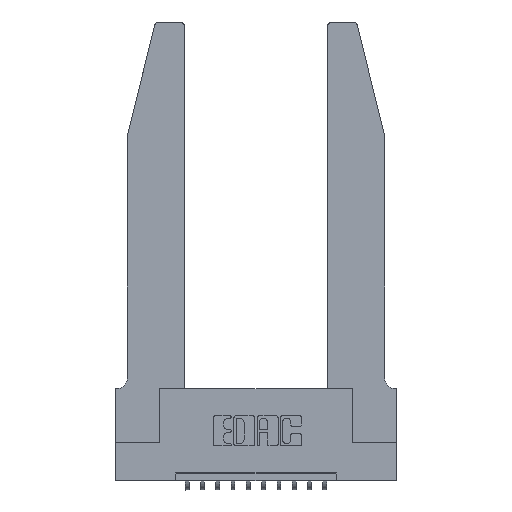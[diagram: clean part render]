
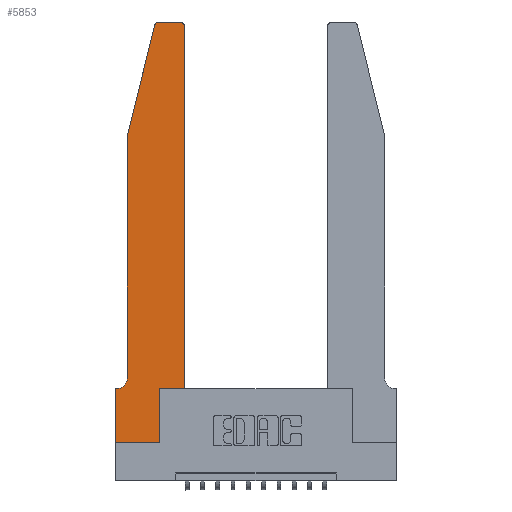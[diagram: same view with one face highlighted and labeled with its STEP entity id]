
A CAD part, top view. The second image highlights one B-rep face of the part: STEP entity #5853.
In plain terms, the highlighted planar face has unit normal (0, 0, 1).
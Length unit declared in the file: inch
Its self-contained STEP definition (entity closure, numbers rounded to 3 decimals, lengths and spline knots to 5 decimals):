
#32 = DIRECTION ( 'NONE',  ( 1., 0., 0. ) ) ;
#38 = ORIENTED_EDGE ( 'NONE', *, *, #14863, .T. ) ;
#209 = VERTEX_POINT ( 'NONE', #15698 ) ;
#236 = PLANE ( 'NONE',  #3552 ) ;
#240 = DIRECTION ( 'NONE',  ( 0., 0., 1. ) ) ;
#488 = CARTESIAN_POINT ( 'NONE',  ( 0.0755, 2., 0.37 ) ) ;
#727 = AXIS2_PLACEMENT_3D ( 'NONE', #13966, #15310, #10030 ) ;
#1046 = EDGE_CURVE ( 'NONE', #7538, #15131, #4470, .T. ) ;
#1056 = ORIENTED_EDGE ( 'NONE', *, *, #11195, .T. ) ;
#1057 = ORIENTED_EDGE ( 'NONE', *, *, #8504, .T. ) ;
#1483 = DIRECTION ( 'NONE',  ( -1., 0., 0. ) ) ;
#1538 = ORIENTED_EDGE ( 'NONE', *, *, #12622, .T. ) ;
#2550 = ORIENTED_EDGE ( 'NONE', *, *, #3011, .T. ) ;
#2638 = DIRECTION ( 'NONE',  ( 0., -1., 0. ) ) ;
#2800 = DIRECTION ( 'NONE',  ( 0., 0., -1. ) ) ;
#2969 = VECTOR ( 'NONE', #8271, 39.37008 ) ;
#3011 = EDGE_CURVE ( 'NONE', #15131, #6401, #12702, .T. ) ;
#3384 = VERTEX_POINT ( 'NONE', #8757 ) ;
#3529 = VECTOR ( 'NONE', #15732, 39.37008 ) ;
#3552 = AXIS2_PLACEMENT_3D ( 'NONE', #10626, #240, #4208 ) ;
#3929 = DIRECTION ( 'NONE',  ( 0., 1., 0. ) ) ;
#3962 = CARTESIAN_POINT ( 'NONE',  ( 0.4205, 2.75, 0.37 ) ) ;
#4182 = CARTESIAN_POINT ( 'NONE',  ( 0., 0., 0.37 ) ) ;
#4208 = DIRECTION ( 'NONE',  ( 1., 0., 0. ) ) ;
#4231 = CARTESIAN_POINT ( 'NONE',  ( 0.25487, 2.72718, 0.37 ) ) ;
#4266 = VECTOR ( 'NONE', #9785, 39.37008 ) ;
#4470 = LINE ( 'NONE', #8400, #4266 ) ;
#4606 = DIRECTION ( 'NONE',  ( 0., -1., 0. ) ) ;
#5055 = ORIENTED_EDGE ( 'NONE', *, *, #6275, .T. ) ;
#5202 = CARTESIAN_POINT ( 'NONE',  ( 0.4205, 2.72, 0.37 ) ) ;
#5614 = CARTESIAN_POINT ( 'NONE',  ( 0.284, 2.75, 0.37 ) ) ;
#5672 = DIRECTION ( 'NONE',  ( -0.239, -0.971, 0. ) ) ;
#5853 = ADVANCED_FACE ( 'NONE', ( #15556 ), #236, .T. ) ;
#5855 = VERTEX_POINT ( 'NONE', #13313 ) ;
#5894 = CARTESIAN_POINT ( 'NONE',  ( 0.0055, 0.35, 0.37 ) ) ;
#5987 = EDGE_CURVE ( 'NONE', #13881, #9811, #12895, .T. ) ;
#6173 = EDGE_CURVE ( 'NONE', #6401, #13881, #13934, .T. ) ;
#6275 = EDGE_CURVE ( 'NONE', #209, #5855, #8270, .T. ) ;
#6278 = EDGE_CURVE ( 'NONE', #13497, #12828, #12287, .T. ) ;
#6327 = VERTEX_POINT ( 'NONE', #5894 ) ;
#6401 = VERTEX_POINT ( 'NONE', #4231 ) ;
#6604 = DIRECTION ( 'NONE',  ( -1., 0., 0. ) ) ;
#7230 = ORIENTED_EDGE ( 'NONE', *, *, #6173, .T. ) ;
#7538 = VERTEX_POINT ( 'NONE', #3962 ) ;
#7610 = CARTESIAN_POINT ( 'NONE',  ( 0.4505, 0.35, 0.37 ) ) ;
#7683 = AXIS2_PLACEMENT_3D ( 'NONE', #10397, #2800, #6604 ) ;
#7750 = LINE ( 'NONE', #13047, #14407 ) ;
#7888 = ORIENTED_EDGE ( 'NONE', *, *, #6278, .T. ) ;
#8023 = CARTESIAN_POINT ( 'NONE',  ( 0.0755, 0.42, 0.37 ) ) ;
#8270 = LINE ( 'NONE', #9878, #13723 ) ;
#8271 = DIRECTION ( 'NONE',  ( 0., 1., 0. ) ) ;
#8400 = CARTESIAN_POINT ( 'NONE',  ( 0.2605, 2.75, 0.37 ) ) ;
#8429 = EDGE_CURVE ( 'NONE', #9811, #6327, #14061, .T. ) ;
#8504 = EDGE_CURVE ( 'NONE', #12828, #3384, #10376, .T. ) ;
#8757 = CARTESIAN_POINT ( 'NONE',  ( 0.2865, 0., 0.37 ) ) ;
#9197 = ORIENTED_EDGE ( 'NONE', *, *, #8429, .T. ) ;
#9221 = CARTESIAN_POINT ( 'NONE',  ( 0.4505, 2.72, 0.37 ) ) ;
#9785 = DIRECTION ( 'NONE',  ( -1., 0., 0. ) ) ;
#9811 = VERTEX_POINT ( 'NONE', #8023 ) ;
#9878 = CARTESIAN_POINT ( 'NONE',  ( 0.4505, 0.35, 0.37 ) ) ;
#9953 = CARTESIAN_POINT ( 'NONE',  ( 0.0755, 2., 0.37 ) ) ;
#10030 = DIRECTION ( 'NONE',  ( 1., 0., 0. ) ) ;
#10376 = LINE ( 'NONE', #4182, #3529 ) ;
#10397 = CARTESIAN_POINT ( 'NONE',  ( 0.0055, 0.42, 0.37 ) ) ;
#10521 = CARTESIAN_POINT ( 'NONE',  ( 0., 0.35, 0.37 ) ) ;
#10626 = CARTESIAN_POINT ( 'NONE',  ( 0., 0.35, 0.37 ) ) ;
#10762 = CIRCLE ( 'NONE', #13118, 0.03 ) ;
#11070 = VECTOR ( 'NONE', #5672, 39.37008 ) ;
#11195 = EDGE_CURVE ( 'NONE', #3384, #209, #16701, .T. ) ;
#11609 = VECTOR ( 'NONE', #3929, 39.37008 ) ;
#11890 = VECTOR ( 'NONE', #2638, 39.37008 ) ;
#12287 = LINE ( 'NONE', #13857, #13096 ) ;
#12554 = DIRECTION ( 'NONE',  ( 1., 0., 0. ) ) ;
#12622 = EDGE_CURVE ( 'NONE', #5855, #13480, #14071, .T. ) ;
#12702 = CIRCLE ( 'NONE', #727, 0.03 ) ;
#12828 = VERTEX_POINT ( 'NONE', #16445 ) ;
#12895 = LINE ( 'NONE', #15472, #11890 ) ;
#13047 = CARTESIAN_POINT ( 'NONE',  ( 0.0755, 0.35, 0.37 ) ) ;
#13096 = VECTOR ( 'NONE', #4606, 39.37008 ) ;
#13118 = AXIS2_PLACEMENT_3D ( 'NONE', #5202, #14344, #32 ) ;
#13221 = ORIENTED_EDGE ( 'NONE', *, *, #1046, .T. ) ;
#13313 = CARTESIAN_POINT ( 'NONE',  ( 0.4505, 0.35, 0.37 ) ) ;
#13430 = EDGE_CURVE ( 'NONE', #13480, #7538, #10762, .T. ) ;
#13480 = VERTEX_POINT ( 'NONE', #9221 ) ;
#13497 = VERTEX_POINT ( 'NONE', #10521 ) ;
#13723 = VECTOR ( 'NONE', #12554, 39.37008 ) ;
#13857 = CARTESIAN_POINT ( 'NONE',  ( 0., 0., 0.37 ) ) ;
#13881 = VERTEX_POINT ( 'NONE', #9953 ) ;
#13934 = LINE ( 'NONE', #488, #11070 ) ;
#13966 = CARTESIAN_POINT ( 'NONE',  ( 0.284, 2.72, 0.37 ) ) ;
#14061 = CIRCLE ( 'NONE', #7683, 0.07 ) ;
#14071 = LINE ( 'NONE', #7610, #11609 ) ;
#14344 = DIRECTION ( 'NONE',  ( 0., 0., 1. ) ) ;
#14407 = VECTOR ( 'NONE', #1483, 39.37008 ) ;
#14602 = ORIENTED_EDGE ( 'NONE', *, *, #5987, .T. ) ;
#14764 = CARTESIAN_POINT ( 'NONE',  ( 0.2865, 0.35, 0.37 ) ) ;
#14863 = EDGE_CURVE ( 'NONE', #6327, #13497, #7750, .T. ) ;
#14882 = EDGE_LOOP ( 'NONE', ( #13221, #2550, #7230, #14602, #9197, #38, #7888, #1057, #1056, #5055, #1538, #15296 ) ) ;
#15131 = VERTEX_POINT ( 'NONE', #5614 ) ;
#15296 = ORIENTED_EDGE ( 'NONE', *, *, #13430, .T. ) ;
#15310 = DIRECTION ( 'NONE',  ( 0., 0., 1. ) ) ;
#15472 = CARTESIAN_POINT ( 'NONE',  ( 0.0755, 2., 0.37 ) ) ;
#15556 = FACE_OUTER_BOUND ( 'NONE', #14882, .T. ) ;
#15698 = CARTESIAN_POINT ( 'NONE',  ( 0.2865, 0.35, 0.37 ) ) ;
#15732 = DIRECTION ( 'NONE',  ( 1., 0., 0. ) ) ;
#16445 = CARTESIAN_POINT ( 'NONE',  ( 0., 0., 0.37 ) ) ;
#16701 = LINE ( 'NONE', #14764, #2969 ) ;
